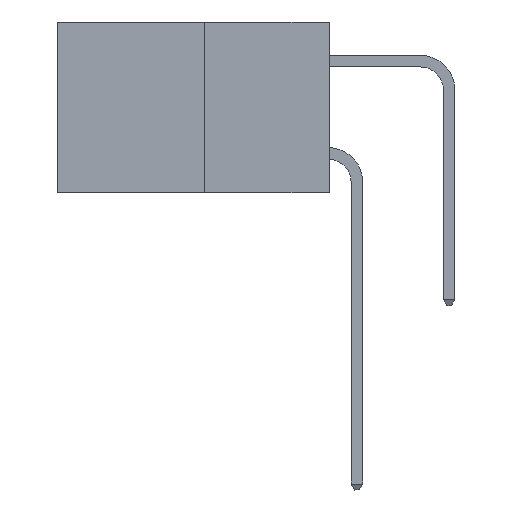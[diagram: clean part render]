
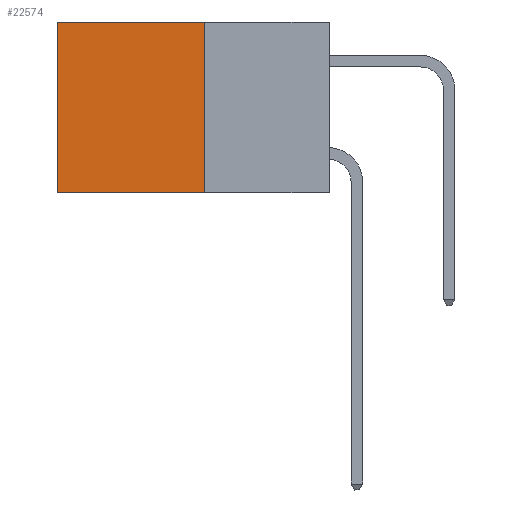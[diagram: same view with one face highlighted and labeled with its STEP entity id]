
A CAD part, left-side view. The second image highlights one B-rep face of the part: STEP entity #22574.
In plain terms, the highlighted planar face has unit normal (-1, 0, 0).
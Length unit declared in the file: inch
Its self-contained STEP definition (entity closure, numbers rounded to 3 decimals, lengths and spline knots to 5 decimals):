
#500 = CARTESIAN_POINT ( 'NONE',  ( 0.277, 0.27, 0. ) ) ;
#722 = DIRECTION ( 'NONE',  ( 0., 0., -1. ) ) ;
#1080 = PLANE ( 'NONE',  #32573 ) ;
#2839 = ORIENTED_EDGE ( 'NONE', *, *, #12331, .F. ) ;
#3315 = LINE ( 'NONE', #8623, #17261 ) ;
#3352 = EDGE_CURVE ( 'NONE', #11506, #29692, #9794, .T. ) ;
#3934 = DIRECTION ( 'NONE',  ( 0., 0., -1. ) ) ;
#4109 = DIRECTION ( 'NONE',  ( 0., 1., 0. ) ) ;
#4765 = CARTESIAN_POINT ( 'NONE',  ( 0.277, 0.59, -0.37 ) ) ;
#6635 = CARTESIAN_POINT ( 'NONE',  ( 0.277, 0.27, -0.37 ) ) ;
#6723 = EDGE_CURVE ( 'NONE', #29692, #23577, #3315, .T. ) ;
#8623 = CARTESIAN_POINT ( 'NONE',  ( 0.277, 0.59, -0.37 ) ) ;
#9794 = LINE ( 'NONE', #24771, #23374 ) ;
#10150 = FACE_OUTER_BOUND ( 'NONE', #11259, .T. ) ;
#11259 = EDGE_LOOP ( 'NONE', ( #19741, #2839, #20422, #28059 ) ) ;
#11506 = VERTEX_POINT ( 'NONE', #500 ) ;
#12331 = EDGE_CURVE ( 'NONE', #19415, #23577, #33652, .T. ) ;
#15713 = DIRECTION ( 'NONE',  ( 0., 1., 0. ) ) ;
#16313 = DIRECTION ( 'NONE',  ( 0., 0., -1. ) ) ;
#16590 = LINE ( 'NONE', #26844, #22063 ) ;
#17261 = VECTOR ( 'NONE', #722, 39.37008 ) ;
#18408 = CARTESIAN_POINT ( 'NONE',  ( 0.277, 0.59, 0. ) ) ;
#19415 = VERTEX_POINT ( 'NONE', #30732 ) ;
#19741 = ORIENTED_EDGE ( 'NONE', *, *, #6723, .T. ) ;
#20422 = ORIENTED_EDGE ( 'NONE', *, *, #34130, .F. ) ;
#20544 = DIRECTION ( 'NONE',  ( 1., 0., 0. ) ) ;
#22063 = VECTOR ( 'NONE', #16313, 39.37008 ) ;
#22574 = ADVANCED_FACE ( 'NONE', ( #10150 ), #1080, .F. ) ;
#23374 = VECTOR ( 'NONE', #4109, 39.37008 ) ;
#23577 = VERTEX_POINT ( 'NONE', #4765 ) ;
#24771 = CARTESIAN_POINT ( 'NONE',  ( 0.277, 0.27, 0. ) ) ;
#26844 = CARTESIAN_POINT ( 'NONE',  ( 0.277, 0.27, -0.37 ) ) ;
#28059 = ORIENTED_EDGE ( 'NONE', *, *, #3352, .T. ) ;
#28873 = CARTESIAN_POINT ( 'NONE',  ( 0.277, 0.27, -0.37 ) ) ;
#29692 = VERTEX_POINT ( 'NONE', #18408 ) ;
#30732 = CARTESIAN_POINT ( 'NONE',  ( 0.277, 0.27, -0.37 ) ) ;
#32573 = AXIS2_PLACEMENT_3D ( 'NONE', #6635, #20544, #3934 ) ;
#32865 = VECTOR ( 'NONE', #15713, 39.37008 ) ;
#33652 = LINE ( 'NONE', #28873, #32865 ) ;
#34130 = EDGE_CURVE ( 'NONE', #11506, #19415, #16590, .T. ) ;
